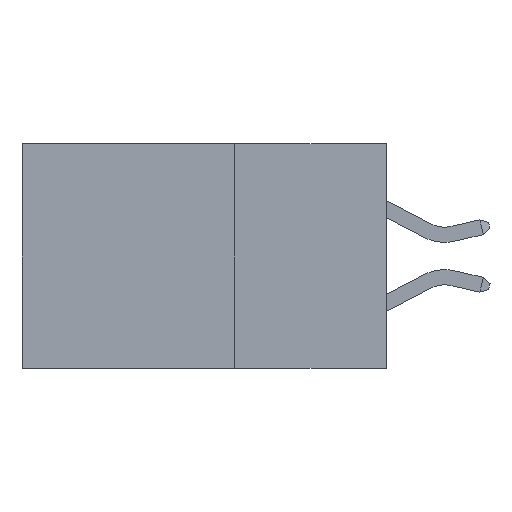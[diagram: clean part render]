
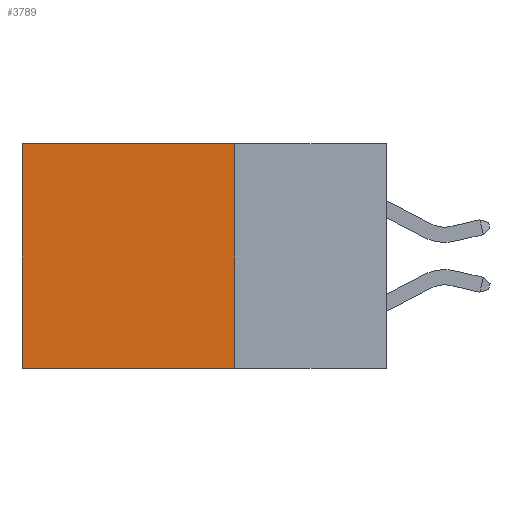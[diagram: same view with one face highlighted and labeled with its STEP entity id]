
A CAD part, left-side view. The second image highlights one B-rep face of the part: STEP entity #3789.
In plain terms, the highlighted planar face has unit normal (-1, 0, 0).
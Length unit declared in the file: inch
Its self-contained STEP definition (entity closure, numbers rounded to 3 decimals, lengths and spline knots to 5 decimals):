
#199 = LINE ( 'NONE', #6778, #5847 ) ;
#744 = ORIENTED_EDGE ( 'NONE', *, *, #2434, .T. ) ;
#765 = EDGE_LOOP ( 'NONE', ( #744, #7004, #4742, #6555 ) ) ;
#1856 = DIRECTION ( 'NONE',  ( 0., 1., 0. ) ) ;
#2434 = EDGE_CURVE ( 'NONE', #21263, #2704, #199, .T. ) ;
#2681 = EDGE_CURVE ( 'NONE', #19583, #2704, #9346, .T. ) ;
#2704 = VERTEX_POINT ( 'NONE', #3770 ) ;
#3291 = VECTOR ( 'NONE', #20625, 39.37008 ) ;
#3686 = VECTOR ( 'NONE', #4312, 39.37008 ) ;
#3770 = CARTESIAN_POINT ( 'NONE',  ( 0.2615, 0.6, -0.37 ) ) ;
#3789 = ADVANCED_FACE ( 'NONE', ( #7237 ), #23092, .F. ) ;
#4312 = DIRECTION ( 'NONE',  ( 0., 0., -1. ) ) ;
#4742 = ORIENTED_EDGE ( 'NONE', *, *, #7503, .F. ) ;
#5847 = VECTOR ( 'NONE', #6810, 39.37008 ) ;
#6555 = ORIENTED_EDGE ( 'NONE', *, *, #9805, .T. ) ;
#6778 = CARTESIAN_POINT ( 'NONE',  ( 0.2615, 0.6, -0.37 ) ) ;
#6810 = DIRECTION ( 'NONE',  ( 0., 0., -1. ) ) ;
#6843 = CARTESIAN_POINT ( 'NONE',  ( 0.2615, 0.25, -0.37 ) ) ;
#7004 = ORIENTED_EDGE ( 'NONE', *, *, #2681, .F. ) ;
#7237 = FACE_OUTER_BOUND ( 'NONE', #765, .T. ) ;
#7503 = EDGE_CURVE ( 'NONE', #11860, #19583, #23020, .T. ) ;
#8008 = CARTESIAN_POINT ( 'NONE',  ( 0.2615, 0.25, 0. ) ) ;
#9346 = LINE ( 'NONE', #19093, #18389 ) ;
#9805 = EDGE_CURVE ( 'NONE', #11860, #21263, #16301, .T. ) ;
#9948 = CARTESIAN_POINT ( 'NONE',  ( 0.2615, 0.25, -0.37 ) ) ;
#11860 = VERTEX_POINT ( 'NONE', #15240 ) ;
#15240 = CARTESIAN_POINT ( 'NONE',  ( 0.2615, 0.25, 0. ) ) ;
#16301 = LINE ( 'NONE', #8008, #3291 ) ;
#16615 = CARTESIAN_POINT ( 'NONE',  ( 0.2615, 0.6, 0. ) ) ;
#18389 = VECTOR ( 'NONE', #1856, 39.37008 ) ;
#19093 = CARTESIAN_POINT ( 'NONE',  ( 0.2615, 0.25, -0.37 ) ) ;
#19583 = VERTEX_POINT ( 'NONE', #6843 ) ;
#20360 = AXIS2_PLACEMENT_3D ( 'NONE', #22681, #22509, #22460 ) ;
#20625 = DIRECTION ( 'NONE',  ( 0., 1., 0. ) ) ;
#21263 = VERTEX_POINT ( 'NONE', #16615 ) ;
#22460 = DIRECTION ( 'NONE',  ( 0., 0., -1. ) ) ;
#22509 = DIRECTION ( 'NONE',  ( 1., 0., 0. ) ) ;
#22681 = CARTESIAN_POINT ( 'NONE',  ( 0.2615, 0.25, -0.37 ) ) ;
#23020 = LINE ( 'NONE', #9948, #3686 ) ;
#23092 = PLANE ( 'NONE',  #20360 ) ;
